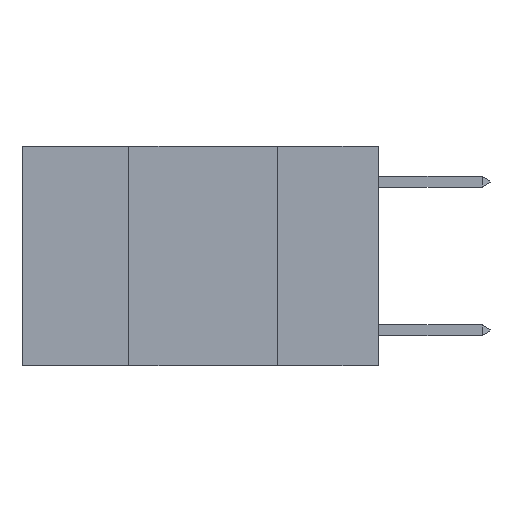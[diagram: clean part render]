
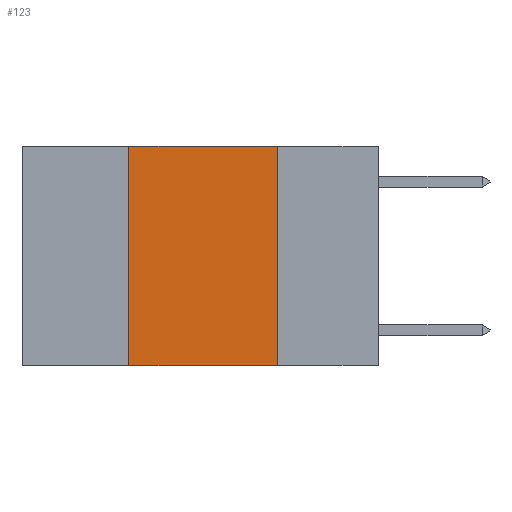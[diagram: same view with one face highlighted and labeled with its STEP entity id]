
A CAD part, left-side view. The second image highlights one B-rep face of the part: STEP entity #123.
In plain terms, the highlighted planar face has unit normal (-1, 0, 0).
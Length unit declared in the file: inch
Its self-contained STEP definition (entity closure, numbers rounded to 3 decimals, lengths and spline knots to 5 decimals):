
#94 = ORIENTED_EDGE ( 'NONE', *, *, #2517, .F. ) ;
#123 = ADVANCED_FACE ( 'NONE', ( #3599 ), #1591, .F. ) ;
#316 = LINE ( 'NONE', #8290, #667 ) ;
#337 = DIRECTION ( 'NONE',  ( 0., -1., 0. ) ) ;
#376 = CARTESIAN_POINT ( 'NONE',  ( 0., 0.6, -0.37 ) ) ;
#510 = VECTOR ( 'NONE', #11151, 39.37008 ) ;
#667 = VECTOR ( 'NONE', #8159, 39.37008 ) ;
#806 = AXIS2_PLACEMENT_3D ( 'NONE', #6860, #10748, #11608 ) ;
#969 = VECTOR ( 'NONE', #337, 39.37008 ) ;
#1159 = LINE ( 'NONE', #11198, #510 ) ;
#1591 = PLANE ( 'NONE',  #806 ) ;
#1954 = ORIENTED_EDGE ( 'NONE', *, *, #4519, .F. ) ;
#2517 = EDGE_CURVE ( 'NONE', #6903, #4341, #1159, .T. ) ;
#3599 = FACE_OUTER_BOUND ( 'NONE', #4473, .T. ) ;
#4341 = VERTEX_POINT ( 'NONE', #8127 ) ;
#4473 = EDGE_LOOP ( 'NONE', ( #1954, #94, #7783, #8040 ) ) ;
#4519 = EDGE_CURVE ( 'NONE', #4341, #13249, #7590, .T. ) ;
#5256 = DIRECTION ( 'NONE',  ( 0., 0., -1. ) ) ;
#5399 = CARTESIAN_POINT ( 'NONE',  ( 0., 0.17, 0. ) ) ;
#5798 = CARTESIAN_POINT ( 'NONE',  ( 0., 0.42, 0. ) ) ;
#6740 = LINE ( 'NONE', #376, #969 ) ;
#6860 = CARTESIAN_POINT ( 'NONE',  ( 0., 0.6, 0. ) ) ;
#6903 = VERTEX_POINT ( 'NONE', #5798 ) ;
#7489 = VECTOR ( 'NONE', #5256, 39.37008 ) ;
#7590 = LINE ( 'NONE', #5399, #7489 ) ;
#7702 = CARTESIAN_POINT ( 'NONE',  ( 0., 0.42, -0.37 ) ) ;
#7783 = ORIENTED_EDGE ( 'NONE', *, *, #9810, .F. ) ;
#8040 = ORIENTED_EDGE ( 'NONE', *, *, #10542, .T. ) ;
#8127 = CARTESIAN_POINT ( 'NONE',  ( 0., 0.17, 0. ) ) ;
#8159 = DIRECTION ( 'NONE',  ( 0., 0., 1. ) ) ;
#8290 = CARTESIAN_POINT ( 'NONE',  ( 0., 0.42, 0. ) ) ;
#9810 = EDGE_CURVE ( 'NONE', #11522, #6903, #316, .T. ) ;
#10542 = EDGE_CURVE ( 'NONE', #11522, #13249, #6740, .T. ) ;
#10625 = CARTESIAN_POINT ( 'NONE',  ( 0., 0.17, -0.37 ) ) ;
#10748 = DIRECTION ( 'NONE',  ( 1., 0., 0. ) ) ;
#11151 = DIRECTION ( 'NONE',  ( 0., -1., 0. ) ) ;
#11198 = CARTESIAN_POINT ( 'NONE',  ( 0., 0.6, 0. ) ) ;
#11522 = VERTEX_POINT ( 'NONE', #7702 ) ;
#11608 = DIRECTION ( 'NONE',  ( 0., 0., -1. ) ) ;
#13249 = VERTEX_POINT ( 'NONE', #10625 ) ;
